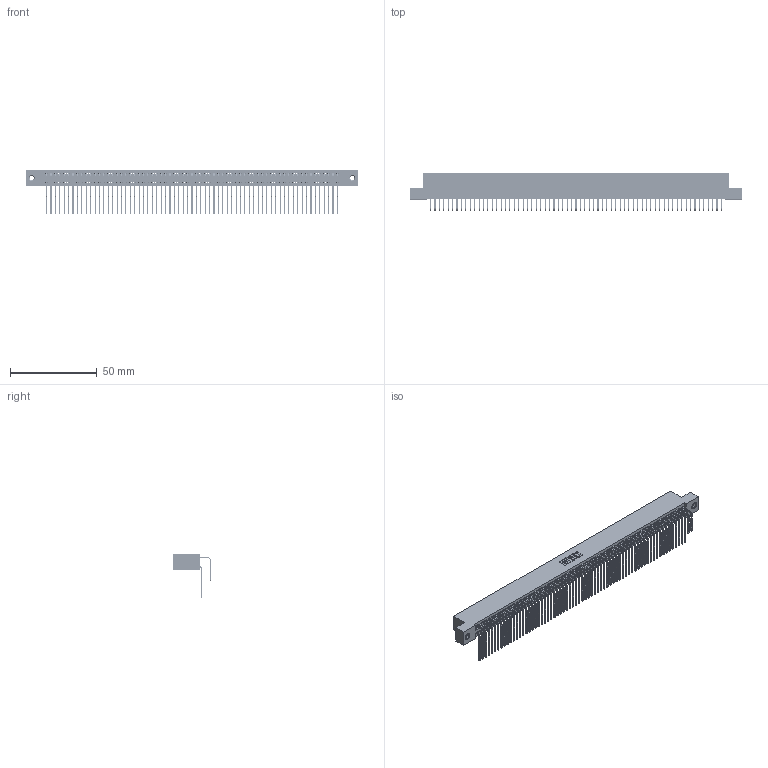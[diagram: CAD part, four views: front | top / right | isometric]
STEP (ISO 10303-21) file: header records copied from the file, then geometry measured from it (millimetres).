
FILE_DESCRIPTION (( 'STEP AP203' ), '1' );
FILE_NAME ('345-134-558-207.STEP', '2018-10-20T10:56:21', ( '' ), ( '' ), 'SwSTEP 2.0', 'SolidWorks 2016', '' );
FILE_SCHEMA (( 'CONFIG_CONTROL_DESIGN' ));
Length unit declared in the file: inch
Products named in the file (5): 345-134-558-207; 345-292-001_558 Tail - 2; 345-292-001_558 559 Tail - 1; 345-250-001_345-250-005-103; 345 Part_Flush Mounting Lugs - 0.156 Dia-TI
Assembly tree (137 placements, depth 2):
  345-134-558-207
    345 Part_Flush Mounting Lugs - 0.156 Dia-TI
    345-292-001_558 559 Tail - 1  x67
    345-292-001_558 Tail - 2  x67
    345-250-001_345-250-005-103  x2
Bounding box: 191.39 x 21.83 x 25.53 mm (x, y, z)
Volume: 19583.3 mm3; surface area: 33094.4 mm2
Topology: 137 solids, 137 shells, 7154 faces, 21247 edges, 13978 vertices
Faces by surface type: plane 4802, cylinder 2336, cone 12, torus 4
Entity records: 52042 total; most frequent: CARTESIAN_POINT 8726, ORIENTED_EDGE 8602, DIRECTION 7663, EDGE_CURVE 4301, VECTOR 3841, LINE 3841, VERTEX_POINT 2860, AXIS2_PLACEMENT_3D 1911
